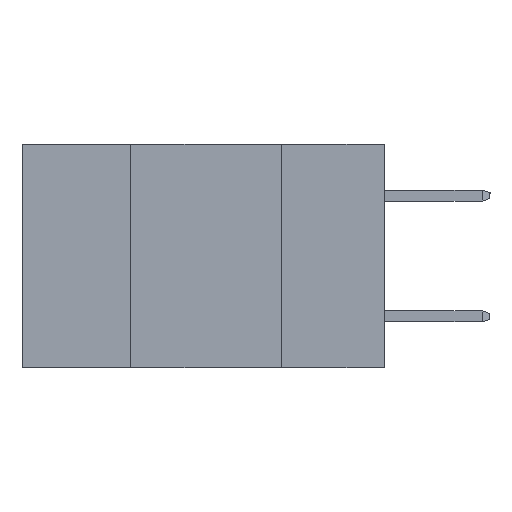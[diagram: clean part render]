
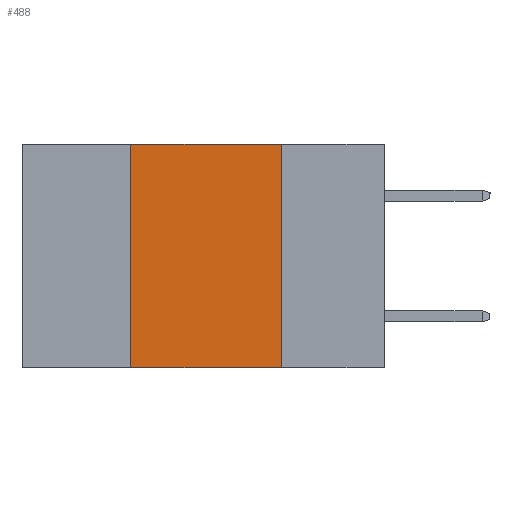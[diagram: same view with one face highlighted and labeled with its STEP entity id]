
A CAD part, left-side view. The second image highlights one B-rep face of the part: STEP entity #488.
In plain terms, the highlighted planar face has unit normal (-1, 0, 0).
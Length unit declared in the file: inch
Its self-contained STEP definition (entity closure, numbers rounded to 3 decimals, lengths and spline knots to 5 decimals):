
#488 = ADVANCED_FACE ( 'NONE', ( #10006 ), #10911, .F. ) ;
#861 = VERTEX_POINT ( 'NONE', #9570 ) ;
#1106 = ORIENTED_EDGE ( 'NONE', *, *, #2622, .F. ) ;
#1190 = CARTESIAN_POINT ( 'NONE',  ( 0., 0.6, -0.37 ) ) ;
#1454 = VECTOR ( 'NONE', #8052, 39.37008 ) ;
#1519 = VERTEX_POINT ( 'NONE', #9213 ) ;
#1651 = DIRECTION ( 'NONE',  ( 0., 0., -1. ) ) ;
#1735 = LINE ( 'NONE', #2735, #8521 ) ;
#2460 = DIRECTION ( 'NONE',  ( 0., -1., 0. ) ) ;
#2546 = VECTOR ( 'NONE', #2460, 39.37008 ) ;
#2599 = CARTESIAN_POINT ( 'NONE',  ( 0., 0.42, -0.37 ) ) ;
#2622 = EDGE_CURVE ( 'NONE', #861, #3699, #1735, .T. ) ;
#2673 = EDGE_LOOP ( 'NONE', ( #1106, #3202, #6508, #7412 ) ) ;
#2735 = CARTESIAN_POINT ( 'NONE',  ( 0., 0.17, -0.37 ) ) ;
#3005 = CARTESIAN_POINT ( 'NONE',  ( 0., 0.17, -0.37 ) ) ;
#3202 = ORIENTED_EDGE ( 'NONE', *, *, #3388, .F. ) ;
#3388 = EDGE_CURVE ( 'NONE', #1519, #861, #11745, .T. ) ;
#3543 = DIRECTION ( 'NONE',  ( 1., 0., 0. ) ) ;
#3699 = VERTEX_POINT ( 'NONE', #3005 ) ;
#4280 = CARTESIAN_POINT ( 'NONE',  ( 0., 0.6, 0. ) ) ;
#4347 = LINE ( 'NONE', #2599, #1454 ) ;
#6508 = ORIENTED_EDGE ( 'NONE', *, *, #6901, .F. ) ;
#6901 = EDGE_CURVE ( 'NONE', #9353, #1519, #4347, .T. ) ;
#7412 = ORIENTED_EDGE ( 'NONE', *, *, #9933, .T. ) ;
#7640 = CARTESIAN_POINT ( 'NONE',  ( 0., 0.42, -0.37 ) ) ;
#8006 = DIRECTION ( 'NONE',  ( 0., 0., -1. ) ) ;
#8052 = DIRECTION ( 'NONE',  ( 0., 0., 1. ) ) ;
#8521 = VECTOR ( 'NONE', #8006, 39.37008 ) ;
#9009 = CARTESIAN_POINT ( 'NONE',  ( 0., 0.6, 0. ) ) ;
#9213 = CARTESIAN_POINT ( 'NONE',  ( 0., 0.42, 0. ) ) ;
#9353 = VERTEX_POINT ( 'NONE', #7640 ) ;
#9355 = AXIS2_PLACEMENT_3D ( 'NONE', #9009, #3543, #1651 ) ;
#9529 = LINE ( 'NONE', #1190, #11389 ) ;
#9570 = CARTESIAN_POINT ( 'NONE',  ( 0., 0.17, 0. ) ) ;
#9710 = DIRECTION ( 'NONE',  ( 0., -1., 0. ) ) ;
#9933 = EDGE_CURVE ( 'NONE', #9353, #3699, #9529, .T. ) ;
#10006 = FACE_OUTER_BOUND ( 'NONE', #2673, .T. ) ;
#10911 = PLANE ( 'NONE',  #9355 ) ;
#11389 = VECTOR ( 'NONE', #9710, 39.37008 ) ;
#11745 = LINE ( 'NONE', #4280, #2546 ) ;
